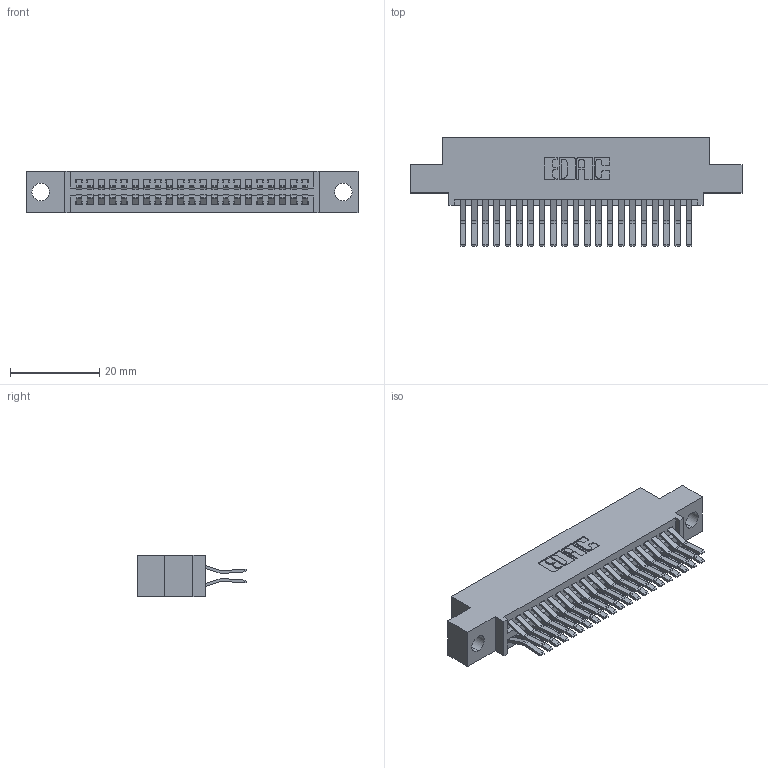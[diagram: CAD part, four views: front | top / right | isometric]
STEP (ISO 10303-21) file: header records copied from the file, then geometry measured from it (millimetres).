
FILE_DESCRIPTION (( 'STEP AP203' ), '1' );
FILE_NAME ('395-042-560-504.STEP', '2018-11-15T13:52:16', ( '' ), ( '' ), 'SwSTEP 2.0', 'SolidWorks 2016', '' );
FILE_SCHEMA (( 'CONFIG_CONTROL_DESIGN' ));
Length unit declared in the file: inch
Products named in the file (3): 345 Part_0.110 Offset - 0.156 Dia-TH; 395-042-560-504; 345-292-001_560 Tail
Assembly tree (43 placements, depth 2):
  395-042-560-504
    345 Part_0.110 Offset - 0.156 Dia-TH
    345-292-001_560 Tail  x42
Bounding box: 74.55 x 24.45 x 9.4 mm (x, y, z)
Volume: 7160.9 mm3; surface area: 10794.3 mm2
Topology: 43 solids, 43 shells, 2314 faces, 6863 edges, 4518 vertices
Faces by surface type: plane 1470, cylinder 844
Entity records: 19527 total; most frequent: CARTESIAN_POINT 3296, ORIENTED_EDGE 3230, DIRECTION 2935, EDGE_CURVE 1615, VECTOR 1395, LINE 1395, VERTEX_POINT 1074, AXIS2_PLACEMENT_3D 770
